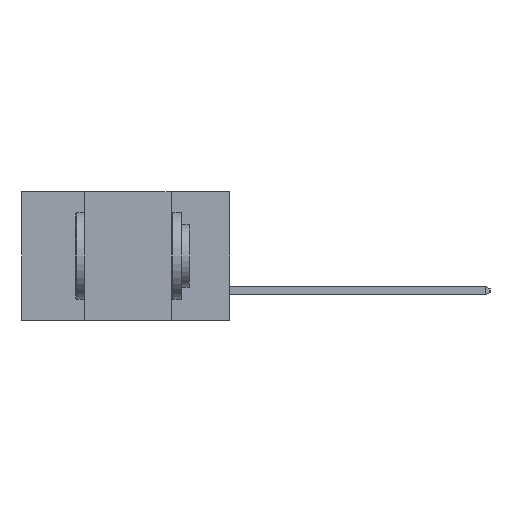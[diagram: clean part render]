
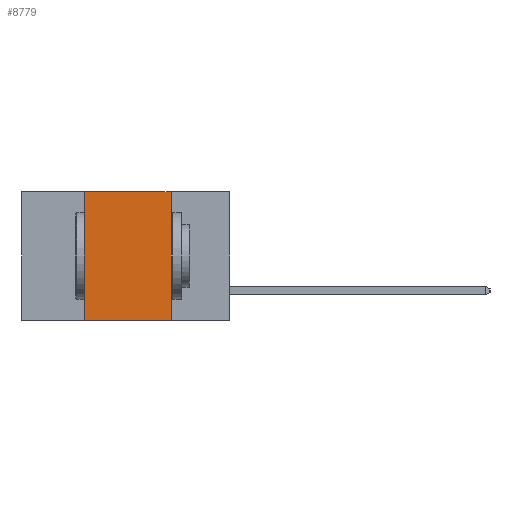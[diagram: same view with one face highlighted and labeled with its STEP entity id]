
A CAD part, left-side view. The second image highlights one B-rep face of the part: STEP entity #8779.
In plain terms, the highlighted planar face has unit normal (-1, 0, 0).
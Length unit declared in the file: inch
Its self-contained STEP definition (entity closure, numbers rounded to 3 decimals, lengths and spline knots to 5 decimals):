
#521 = LINE ( 'NONE', #4681, #1002 ) ;
#633 = CARTESIAN_POINT ( 'NONE',  ( 0., 0.17, -0.37 ) ) ;
#1002 = VECTOR ( 'NONE', #6172, 39.37008 ) ;
#1689 = ORIENTED_EDGE ( 'NONE', *, *, #6182, .F. ) ;
#1897 = ORIENTED_EDGE ( 'NONE', *, *, #8201, .F. ) ;
#2349 = ORIENTED_EDGE ( 'NONE', *, *, #14805, .F. ) ;
#2375 = DIRECTION ( 'NONE',  ( 0., 0., -1. ) ) ;
#2398 = DIRECTION ( 'NONE',  ( 1., 0., 0. ) ) ;
#2749 = ORIENTED_EDGE ( 'NONE', *, *, #16991, .T. ) ;
#2764 = PLANE ( 'NONE',  #10850 ) ;
#3025 = EDGE_LOOP ( 'NONE', ( #1689, #2349, #1897, #2749 ) ) ;
#4317 = DIRECTION ( 'NONE',  ( 0., 0., 1. ) ) ;
#4681 = CARTESIAN_POINT ( 'NONE',  ( 0., 0.6, -0.37 ) ) ;
#6147 = CARTESIAN_POINT ( 'NONE',  ( 0., 0.42, 0. ) ) ;
#6172 = DIRECTION ( 'NONE',  ( 0., -1., 0. ) ) ;
#6182 = EDGE_CURVE ( 'NONE', #6511, #8946, #12283, .T. ) ;
#6206 = CARTESIAN_POINT ( 'NONE',  ( 0., 0.6, 0. ) ) ;
#6511 = VERTEX_POINT ( 'NONE', #15365 ) ;
#8201 = EDGE_CURVE ( 'NONE', #9704, #15439, #16272, .T. ) ;
#8277 = CARTESIAN_POINT ( 'NONE',  ( 0., 0.42, 0. ) ) ;
#8514 = VECTOR ( 'NONE', #4317, 39.37008 ) ;
#8779 = ADVANCED_FACE ( 'NONE', ( #9168 ), #2764, .F. ) ;
#8946 = VERTEX_POINT ( 'NONE', #633 ) ;
#9168 = FACE_OUTER_BOUND ( 'NONE', #3025, .T. ) ;
#9704 = VERTEX_POINT ( 'NONE', #10374 ) ;
#10262 = LINE ( 'NONE', #18458, #18401 ) ;
#10374 = CARTESIAN_POINT ( 'NONE',  ( 0., 0.42, -0.37 ) ) ;
#10850 = AXIS2_PLACEMENT_3D ( 'NONE', #6206, #2398, #2375 ) ;
#12283 = LINE ( 'NONE', #15345, #15648 ) ;
#14805 = EDGE_CURVE ( 'NONE', #15439, #6511, #10262, .T. ) ;
#15345 = CARTESIAN_POINT ( 'NONE',  ( 0., 0.17, 0. ) ) ;
#15365 = CARTESIAN_POINT ( 'NONE',  ( 0., 0.17, 0. ) ) ;
#15439 = VERTEX_POINT ( 'NONE', #8277 ) ;
#15601 = DIRECTION ( 'NONE',  ( 0., -1., 0. ) ) ;
#15648 = VECTOR ( 'NONE', #18266, 39.37008 ) ;
#16272 = LINE ( 'NONE', #6147, #8514 ) ;
#16991 = EDGE_CURVE ( 'NONE', #9704, #8946, #521, .T. ) ;
#18266 = DIRECTION ( 'NONE',  ( 0., 0., -1. ) ) ;
#18401 = VECTOR ( 'NONE', #15601, 39.37008 ) ;
#18458 = CARTESIAN_POINT ( 'NONE',  ( 0., 0.6, 0. ) ) ;
